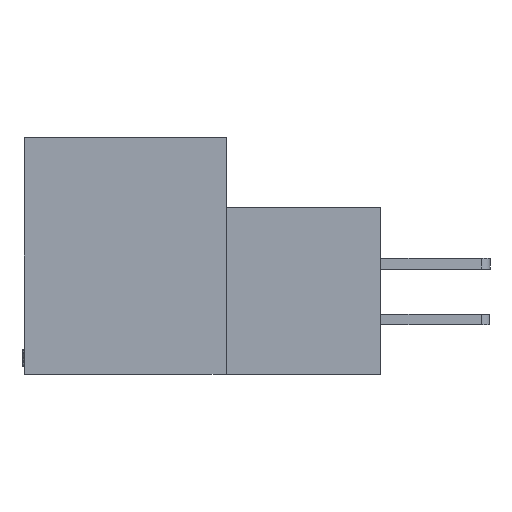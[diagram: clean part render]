
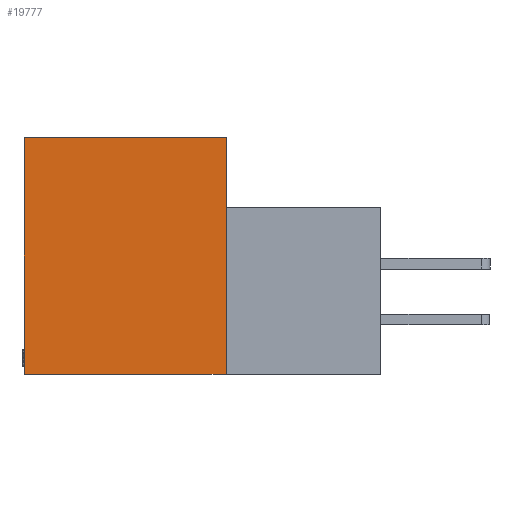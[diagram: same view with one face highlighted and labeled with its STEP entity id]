
A CAD part, left-side view. The second image highlights one B-rep face of the part: STEP entity #19777.
In plain terms, the highlighted planar face has unit normal (-1, 0, 0).
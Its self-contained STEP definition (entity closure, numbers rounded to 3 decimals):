
#908 = VERTEX_POINT ( 'NONE', #10092 ) ;
#934 = AXIS2_PLACEMENT_3D ( 'NONE', #16525, #5420, #3480 ) ;
#1778 = ORIENTED_EDGE ( 'NONE', *, *, #4117, .F. ) ;
#2000 = EDGE_CURVE ( 'NONE', #21172, #16233, #18357, .T. ) ;
#2736 = CARTESIAN_POINT ( 'NONE',  ( 0., 0., -13.487 ) ) ;
#2930 = VECTOR ( 'NONE', #7773, 1000. ) ;
#3480 = DIRECTION ( 'NONE',  ( 0., 0., -1. ) ) ;
#3737 = CARTESIAN_POINT ( 'NONE',  ( 0., -8.814, -13.487 ) ) ;
#3977 = DIRECTION ( 'NONE',  ( 0., -1., 0. ) ) ;
#4117 = EDGE_CURVE ( 'NONE', #7222, #908, #23507, .T. ) ;
#5420 = DIRECTION ( 'NONE',  ( 1., 0., 0. ) ) ;
#7222 = VERTEX_POINT ( 'NONE', #23817 ) ;
#7773 = DIRECTION ( 'NONE',  ( 0., 1., 0. ) ) ;
#8538 = ORIENTED_EDGE ( 'NONE', *, *, #15609, .F. ) ;
#9105 = CARTESIAN_POINT ( 'NONE',  ( 0., 11.506, -13.487 ) ) ;
#10092 = CARTESIAN_POINT ( 'NONE',  ( 0., 11.506, 0. ) ) ;
#11596 = VECTOR ( 'NONE', #3977, 1000. ) ;
#15549 = EDGE_CURVE ( 'NONE', #16233, #7222, #21777, .T. ) ;
#15609 = EDGE_CURVE ( 'NONE', #908, #21172, #17720, .T. ) ;
#16233 = VERTEX_POINT ( 'NONE', #2736 ) ;
#16525 = CARTESIAN_POINT ( 'NONE',  ( 0., 0., 0. ) ) ;
#16862 = ORIENTED_EDGE ( 'NONE', *, *, #15549, .F. ) ;
#16865 = CARTESIAN_POINT ( 'NONE',  ( 0., 11.506, 0. ) ) ;
#17720 = LINE ( 'NONE', #16865, #11596 ) ;
#18244 = EDGE_LOOP ( 'NONE', ( #16862, #21251, #8538, #1778 ) ) ;
#18357 = LINE ( 'NONE', #19022, #20669 ) ;
#18573 = VECTOR ( 'NONE', #20127, 1000. ) ;
#18938 = DIRECTION ( 'NONE',  ( 0., 0., -1. ) ) ;
#19022 = CARTESIAN_POINT ( 'NONE',  ( 0., 0., 0. ) ) ;
#19131 = CARTESIAN_POINT ( 'NONE',  ( 0., 0., 0. ) ) ;
#19777 = ADVANCED_FACE ( 'NONE', ( #21032 ), #20030, .F. ) ;
#20030 = PLANE ( 'NONE',  #934 ) ;
#20127 = DIRECTION ( 'NONE',  ( 0., 0., 1. ) ) ;
#20669 = VECTOR ( 'NONE', #18938, 1000. ) ;
#21032 = FACE_OUTER_BOUND ( 'NONE', #18244, .T. ) ;
#21172 = VERTEX_POINT ( 'NONE', #19131 ) ;
#21251 = ORIENTED_EDGE ( 'NONE', *, *, #2000, .F. ) ;
#21777 = LINE ( 'NONE', #3737, #2930 ) ;
#23507 = LINE ( 'NONE', #9105, #18573 ) ;
#23817 = CARTESIAN_POINT ( 'NONE',  ( 0., 11.506, -13.487 ) ) ;
